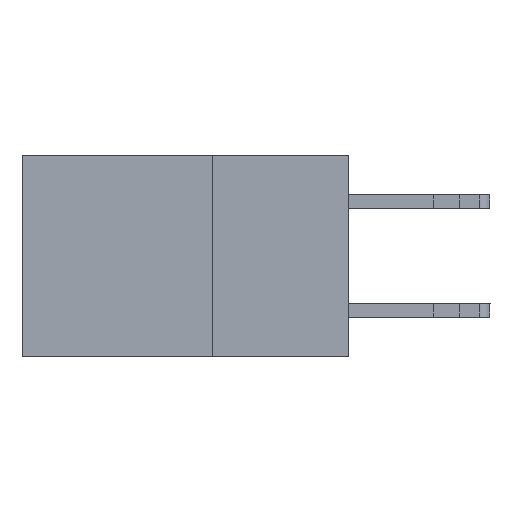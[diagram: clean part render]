
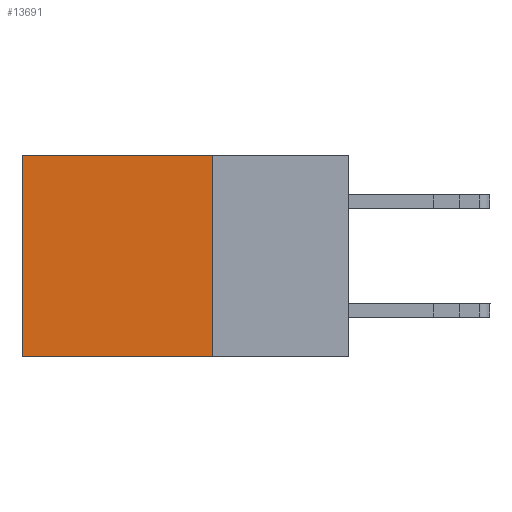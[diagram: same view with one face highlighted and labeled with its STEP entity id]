
A CAD part, left-side view. The second image highlights one B-rep face of the part: STEP entity #13691.
In plain terms, the highlighted planar face has unit normal (-1, 0, 0).
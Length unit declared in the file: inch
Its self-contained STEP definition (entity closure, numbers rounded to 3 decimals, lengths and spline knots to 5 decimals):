
#323 = DIRECTION ( 'NONE',  ( 0., 0., -1. ) ) ;
#1358 = CARTESIAN_POINT ( 'NONE',  ( 0.2615, 0.25, -0.37 ) ) ;
#1609 = VECTOR ( 'NONE', #12275, 39.37008 ) ;
#2086 = EDGE_LOOP ( 'NONE', ( #14825, #18424, #16268, #14647 ) ) ;
#3468 = CARTESIAN_POINT ( 'NONE',  ( 0.2615, 0.25, -0.37 ) ) ;
#4295 = LINE ( 'NONE', #15964, #8361 ) ;
#4302 = EDGE_CURVE ( 'NONE', #14082, #18347, #5680, .T. ) ;
#4458 = PLANE ( 'NONE',  #6439 ) ;
#5680 = LINE ( 'NONE', #12478, #1609 ) ;
#5895 = CARTESIAN_POINT ( 'NONE',  ( 0.2615, 0.25, -0.37 ) ) ;
#5993 = DIRECTION ( 'NONE',  ( 0., 0., -1. ) ) ;
#6396 = LINE ( 'NONE', #5895, #19136 ) ;
#6439 = AXIS2_PLACEMENT_3D ( 'NONE', #1358, #15215, #5993 ) ;
#6444 = LINE ( 'NONE', #18794, #10029 ) ;
#6745 = DIRECTION ( 'NONE',  ( 0., 0., -1. ) ) ;
#8361 = VECTOR ( 'NONE', #6745, 39.37008 ) ;
#8890 = EDGE_CURVE ( 'NONE', #14082, #17297, #4295, .T. ) ;
#9472 = EDGE_CURVE ( 'NONE', #18347, #13428, #6444, .T. ) ;
#10029 = VECTOR ( 'NONE', #323, 39.37008 ) ;
#10032 = CARTESIAN_POINT ( 'NONE',  ( 0.2615, 0.6, -0.37 ) ) ;
#12275 = DIRECTION ( 'NONE',  ( 0., 1., 0. ) ) ;
#12478 = CARTESIAN_POINT ( 'NONE',  ( 0.2615, 0.25, 0. ) ) ;
#13428 = VERTEX_POINT ( 'NONE', #10032 ) ;
#13691 = ADVANCED_FACE ( 'NONE', ( #13725 ), #4458, .F. ) ;
#13725 = FACE_OUTER_BOUND ( 'NONE', #2086, .T. ) ;
#14082 = VERTEX_POINT ( 'NONE', #17912 ) ;
#14647 = ORIENTED_EDGE ( 'NONE', *, *, #4302, .T. ) ;
#14825 = ORIENTED_EDGE ( 'NONE', *, *, #9472, .T. ) ;
#15215 = DIRECTION ( 'NONE',  ( 1., 0., 0. ) ) ;
#15964 = CARTESIAN_POINT ( 'NONE',  ( 0.2615, 0.25, -0.37 ) ) ;
#16268 = ORIENTED_EDGE ( 'NONE', *, *, #8890, .F. ) ;
#16320 = EDGE_CURVE ( 'NONE', #17297, #13428, #6396, .T. ) ;
#16678 = DIRECTION ( 'NONE',  ( 0., 1., 0. ) ) ;
#17297 = VERTEX_POINT ( 'NONE', #3468 ) ;
#17912 = CARTESIAN_POINT ( 'NONE',  ( 0.2615, 0.25, 0. ) ) ;
#18347 = VERTEX_POINT ( 'NONE', #19139 ) ;
#18424 = ORIENTED_EDGE ( 'NONE', *, *, #16320, .F. ) ;
#18794 = CARTESIAN_POINT ( 'NONE',  ( 0.2615, 0.6, -0.37 ) ) ;
#19136 = VECTOR ( 'NONE', #16678, 39.37008 ) ;
#19139 = CARTESIAN_POINT ( 'NONE',  ( 0.2615, 0.6, 0. ) ) ;
